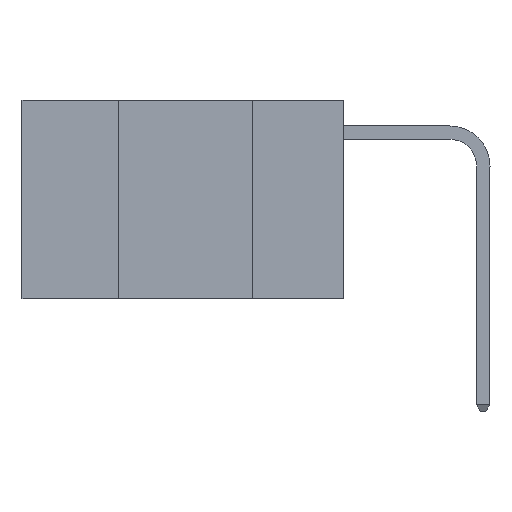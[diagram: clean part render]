
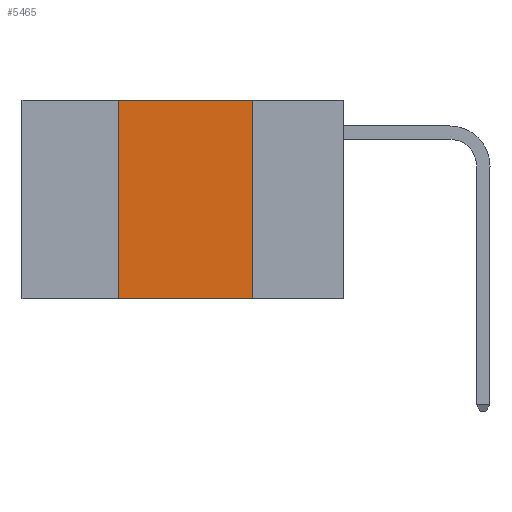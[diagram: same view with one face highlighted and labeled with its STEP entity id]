
A CAD part, left-side view. The second image highlights one B-rep face of the part: STEP entity #5465.
In plain terms, the highlighted planar face has unit normal (-1, 0, 0).
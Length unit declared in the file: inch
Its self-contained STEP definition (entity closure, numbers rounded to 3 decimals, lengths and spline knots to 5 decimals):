
#582 = LINE ( 'NONE', #8403, #2984 ) ;
#586 = VECTOR ( 'NONE', #11103, 39.37008 ) ;
#824 = DIRECTION ( 'NONE',  ( 0., -1., 0. ) ) ;
#875 = ORIENTED_EDGE ( 'NONE', *, *, #7195, .F. ) ;
#905 = LINE ( 'NONE', #4309, #586 ) ;
#1874 = VECTOR ( 'NONE', #1954, 39.37008 ) ;
#1954 = DIRECTION ( 'NONE',  ( 0., 0., 1. ) ) ;
#2580 = PLANE ( 'NONE',  #4386 ) ;
#2713 = ORIENTED_EDGE ( 'NONE', *, *, #7582, .F. ) ;
#2984 = VECTOR ( 'NONE', #9288, 39.37008 ) ;
#3192 = ORIENTED_EDGE ( 'NONE', *, *, #11164, .T. ) ;
#3576 = DIRECTION ( 'NONE',  ( 1., 0., 0. ) ) ;
#3867 = CARTESIAN_POINT ( 'NONE',  ( 0., 0.17, 0. ) ) ;
#4309 = CARTESIAN_POINT ( 'NONE',  ( 0., 0.17, 0. ) ) ;
#4386 = AXIS2_PLACEMENT_3D ( 'NONE', #9528, #3576, #10446 ) ;
#4821 = CARTESIAN_POINT ( 'NONE',  ( 0., 0.42, 0. ) ) ;
#5296 = LINE ( 'NONE', #6103, #1874 ) ;
#5465 = ADVANCED_FACE ( 'NONE', ( #9586 ), #2580, .F. ) ;
#6103 = CARTESIAN_POINT ( 'NONE',  ( 0., 0.42, 0. ) ) ;
#6220 = VERTEX_POINT ( 'NONE', #8750 ) ;
#6652 = CARTESIAN_POINT ( 'NONE',  ( 0., 0.42, -0.37 ) ) ;
#7068 = CARTESIAN_POINT ( 'NONE',  ( 0., 0.6, 0. ) ) ;
#7183 = VERTEX_POINT ( 'NONE', #3867 ) ;
#7195 = EDGE_CURVE ( 'NONE', #9800, #7183, #10526, .T. ) ;
#7582 = EDGE_CURVE ( 'NONE', #7183, #6220, #905, .T. ) ;
#8403 = CARTESIAN_POINT ( 'NONE',  ( 0., 0.6, -0.37 ) ) ;
#8494 = EDGE_CURVE ( 'NONE', #12647, #9800, #5296, .T. ) ;
#8750 = CARTESIAN_POINT ( 'NONE',  ( 0., 0.17, -0.37 ) ) ;
#9288 = DIRECTION ( 'NONE',  ( 0., -1., 0. ) ) ;
#9528 = CARTESIAN_POINT ( 'NONE',  ( 0., 0.6, 0. ) ) ;
#9586 = FACE_OUTER_BOUND ( 'NONE', #11787, .T. ) ;
#9800 = VERTEX_POINT ( 'NONE', #4821 ) ;
#10181 = ORIENTED_EDGE ( 'NONE', *, *, #8494, .F. ) ;
#10446 = DIRECTION ( 'NONE',  ( 0., 0., -1. ) ) ;
#10526 = LINE ( 'NONE', #7068, #12083 ) ;
#11103 = DIRECTION ( 'NONE',  ( 0., 0., -1. ) ) ;
#11164 = EDGE_CURVE ( 'NONE', #12647, #6220, #582, .T. ) ;
#11787 = EDGE_LOOP ( 'NONE', ( #2713, #875, #10181, #3192 ) ) ;
#12083 = VECTOR ( 'NONE', #824, 39.37008 ) ;
#12647 = VERTEX_POINT ( 'NONE', #6652 ) ;
